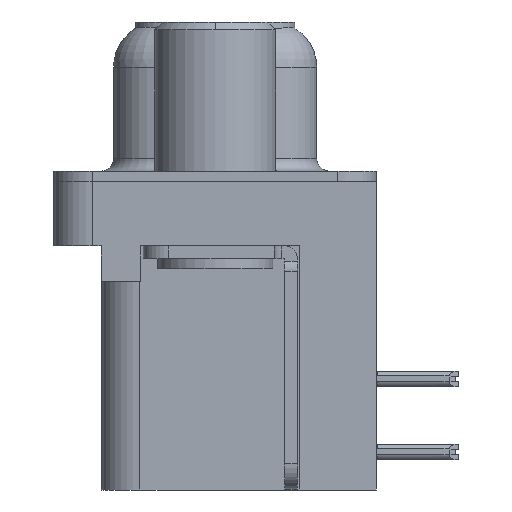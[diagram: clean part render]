
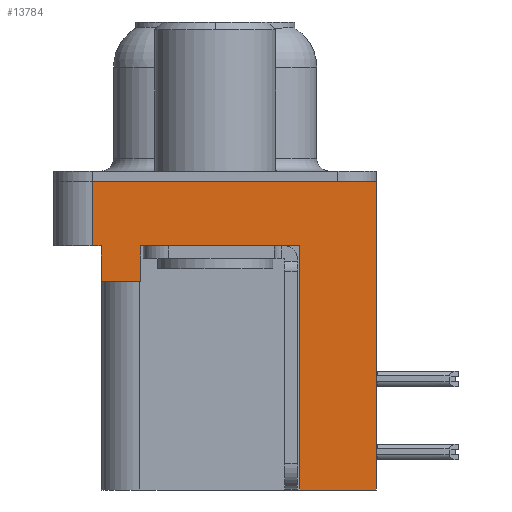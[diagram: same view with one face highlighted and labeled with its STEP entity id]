
A CAD part, left-side view. The second image highlights one B-rep face of the part: STEP entity #13784.
In plain terms, the highlighted planar face has unit normal (-1, 0, 0).
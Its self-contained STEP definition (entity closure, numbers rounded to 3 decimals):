
#683 = ORIENTED_EDGE ( 'NONE', *, *, #19775, .F. ) ;
#788 = CARTESIAN_POINT ( 'NONE',  ( -2.91, -6.275, -2.5 ) ) ;
#902 = LINE ( 'NONE', #3814, #19401 ) ;
#1391 = CARTESIAN_POINT ( 'NONE',  ( -2.91, 4.775, -2.5 ) ) ;
#1457 = DIRECTION ( 'NONE',  ( 0., 1., 0. ) ) ;
#1537 = CARTESIAN_POINT ( 'NONE',  ( -2.91, 4.425, -3.9 ) ) ;
#1554 = DIRECTION ( 'NONE',  ( 0., -1., 0. ) ) ;
#1751 = CARTESIAN_POINT ( 'NONE',  ( -2.91, -3.295, -12. ) ) ;
#1860 = ORIENTED_EDGE ( 'NONE', *, *, #19980, .F. ) ;
#2193 = LINE ( 'NONE', #17331, #9697 ) ;
#2792 = CARTESIAN_POINT ( 'NONE',  ( -2.91, 4.775, -2.5 ) ) ;
#3027 = LINE ( 'NONE', #788, #5364 ) ;
#3395 = EDGE_CURVE ( 'NONE', #12881, #23274, #2193, .T. ) ;
#3694 = DIRECTION ( 'NONE',  ( -1., 0., 0. ) ) ;
#3814 = CARTESIAN_POINT ( 'NONE',  ( -2.91, -6.275, 0. ) ) ;
#4096 = VECTOR ( 'NONE', #16528, 1000. ) ;
#4123 = VERTEX_POINT ( 'NONE', #18198 ) ;
#4350 = EDGE_CURVE ( 'NONE', #15947, #4123, #5244, .T. ) ;
#4399 = LINE ( 'NONE', #22009, #4096 ) ;
#4702 = VECTOR ( 'NONE', #1554, 1000. ) ;
#4954 = VECTOR ( 'NONE', #16286, 1000. ) ;
#5071 = EDGE_CURVE ( 'NONE', #23665, #17893, #4399, .T. ) ;
#5119 = CARTESIAN_POINT ( 'NONE',  ( -2.91, -6.275, -12. ) ) ;
#5244 = LINE ( 'NONE', #2792, #14720 ) ;
#5364 = VECTOR ( 'NONE', #10083, 1000. ) ;
#5520 = LINE ( 'NONE', #1751, #4954 ) ;
#5656 = EDGE_CURVE ( 'NONE', #15733, #16406, #5520, .T. ) ;
#5743 = ORIENTED_EDGE ( 'NONE', *, *, #10127, .T. ) ;
#6099 = CARTESIAN_POINT ( 'NONE',  ( -2.91, 2.895, -2.5 ) ) ;
#6388 = VECTOR ( 'NONE', #14441, 1000. ) ;
#6413 = DIRECTION ( 'NONE',  ( 0., 0., 1. ) ) ;
#6671 = LINE ( 'NONE', #16766, #19672 ) ;
#9392 = DIRECTION ( 'NONE',  ( 0., 0., 1. ) ) ;
#9598 = LINE ( 'NONE', #20226, #4702 ) ;
#9697 = VECTOR ( 'NONE', #21270, 1000. ) ;
#9853 = CARTESIAN_POINT ( 'NONE',  ( -2.91, -3.295, -2.5 ) ) ;
#10083 = DIRECTION ( 'NONE',  ( 0., -1., 0. ) ) ;
#10121 = ORIENTED_EDGE ( 'NONE', *, *, #5071, .T. ) ;
#10127 = EDGE_CURVE ( 'NONE', #17893, #16406, #3027, .T. ) ;
#10915 = CARTESIAN_POINT ( 'NONE',  ( -2.91, -3.295, -12. ) ) ;
#11585 = AXIS2_PLACEMENT_3D ( 'NONE', #18625, #3694, #16625 ) ;
#12221 = VERTEX_POINT ( 'NONE', #17894 ) ;
#12881 = VERTEX_POINT ( 'NONE', #13908 ) ;
#13202 = EDGE_LOOP ( 'NONE', ( #683, #14816, #20498, #13478, #20183, #10121, #5743, #22362, #1860, #18003 ) ) ;
#13478 = ORIENTED_EDGE ( 'NONE', *, *, #3395, .F. ) ;
#13784 = ADVANCED_FACE ( 'NONE', ( #16647 ), #18549, .T. ) ;
#13908 = CARTESIAN_POINT ( 'NONE',  ( -2.91, 4.425, -3.9 ) ) ;
#14441 = DIRECTION ( 'NONE',  ( 0., 1., 0. ) ) ;
#14720 = VECTOR ( 'NONE', #6413, 1000. ) ;
#14816 = ORIENTED_EDGE ( 'NONE', *, *, #4350, .F. ) ;
#14901 = EDGE_CURVE ( 'NONE', #23665, #12881, #19589, .T. ) ;
#15733 = VERTEX_POINT ( 'NONE', #15843 ) ;
#15843 = CARTESIAN_POINT ( 'NONE',  ( -2.91, -3.295, -12. ) ) ;
#15947 = VERTEX_POINT ( 'NONE', #1391 ) ;
#16286 = DIRECTION ( 'NONE',  ( 0., 0., 1. ) ) ;
#16406 = VERTEX_POINT ( 'NONE', #9853 ) ;
#16528 = DIRECTION ( 'NONE',  ( 0., 0., 1. ) ) ;
#16625 = DIRECTION ( 'NONE',  ( 0., 0., 1. ) ) ;
#16647 = FACE_OUTER_BOUND ( 'NONE', #13202, .T. ) ;
#16766 = CARTESIAN_POINT ( 'NONE',  ( -2.91, -6.275, -2.5 ) ) ;
#17331 = CARTESIAN_POINT ( 'NONE',  ( -2.91, 4.425, -3.9 ) ) ;
#17893 = VERTEX_POINT ( 'NONE', #6099 ) ;
#17894 = CARTESIAN_POINT ( 'NONE',  ( -2.91, -6.275, 0. ) ) ;
#18003 = ORIENTED_EDGE ( 'NONE', *, *, #21613, .T. ) ;
#18198 = CARTESIAN_POINT ( 'NONE',  ( -2.91, 4.775, 0. ) ) ;
#18549 = PLANE ( 'NONE',  #11585 ) ;
#18625 = CARTESIAN_POINT ( 'NONE',  ( -2.91, -6.275, -2.5 ) ) ;
#19401 = VECTOR ( 'NONE', #22488, 1000. ) ;
#19589 = LINE ( 'NONE', #1537, #19876 ) ;
#19634 = EDGE_CURVE ( 'NONE', #15947, #23274, #9598, .T. ) ;
#19672 = VECTOR ( 'NONE', #9392, 1000. ) ;
#19775 = EDGE_CURVE ( 'NONE', #4123, #12221, #902, .T. ) ;
#19876 = VECTOR ( 'NONE', #1457, 1000. ) ;
#19980 = EDGE_CURVE ( 'NONE', #22210, #15733, #21719, .T. ) ;
#20183 = ORIENTED_EDGE ( 'NONE', *, *, #14901, .F. ) ;
#20226 = CARTESIAN_POINT ( 'NONE',  ( -2.91, -6.275, -2.5 ) ) ;
#20498 = ORIENTED_EDGE ( 'NONE', *, *, #19634, .T. ) ;
#21270 = DIRECTION ( 'NONE',  ( 0., 0., 1. ) ) ;
#21613 = EDGE_CURVE ( 'NONE', #22210, #12221, #6671, .T. ) ;
#21719 = LINE ( 'NONE', #10915, #6388 ) ;
#21985 = CARTESIAN_POINT ( 'NONE',  ( -2.91, 2.895, -3.9 ) ) ;
#22009 = CARTESIAN_POINT ( 'NONE',  ( -2.91, 2.895, -3.9 ) ) ;
#22210 = VERTEX_POINT ( 'NONE', #5119 ) ;
#22362 = ORIENTED_EDGE ( 'NONE', *, *, #5656, .F. ) ;
#22488 = DIRECTION ( 'NONE',  ( 0., -1., 0. ) ) ;
#22830 = CARTESIAN_POINT ( 'NONE',  ( -2.91, 4.425, -2.5 ) ) ;
#23274 = VERTEX_POINT ( 'NONE', #22830 ) ;
#23665 = VERTEX_POINT ( 'NONE', #21985 ) ;
